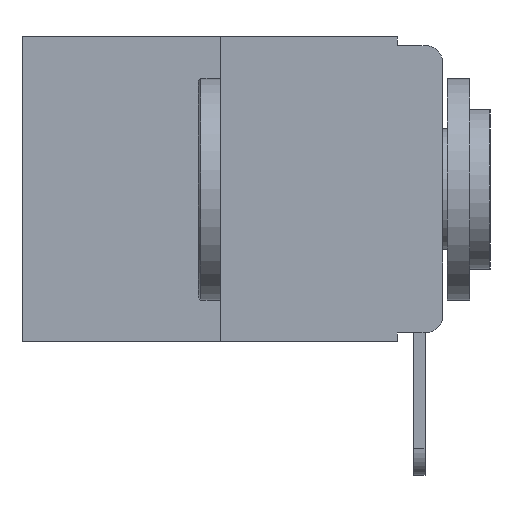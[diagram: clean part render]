
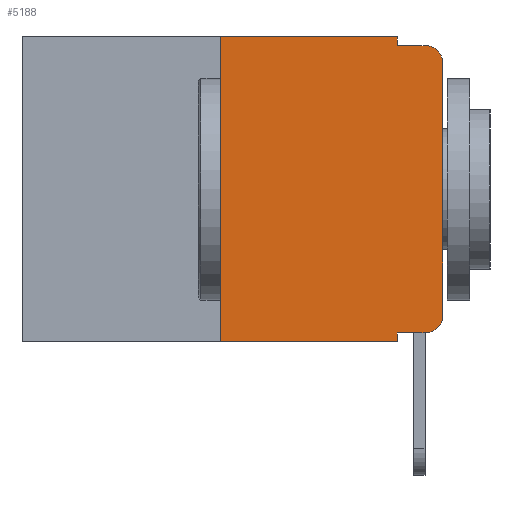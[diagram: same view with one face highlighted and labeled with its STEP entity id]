
A CAD part, left-side view. The second image highlights one B-rep face of the part: STEP entity #5188.
In plain terms, the highlighted planar face has unit normal (-1, 0, 0).
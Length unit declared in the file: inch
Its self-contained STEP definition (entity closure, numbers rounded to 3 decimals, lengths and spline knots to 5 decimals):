
#161 = ORIENTED_EDGE ( 'NONE', *, *, #17154, .T. ) ;
#173 = ORIENTED_EDGE ( 'NONE', *, *, #4821, .T. ) ;
#313 = DIRECTION ( 'NONE',  ( 0., 0., -1. ) ) ;
#349 = CARTESIAN_POINT ( 'NONE',  ( 0., 0.051, -0.343 ) ) ;
#486 = CARTESIAN_POINT ( 'NONE',  ( 0., 0.02, -0.01 ) ) ;
#583 = VECTOR ( 'NONE', #7805, 39.37008 ) ;
#1150 = ORIENTED_EDGE ( 'NONE', *, *, #4353, .F. ) ;
#1375 = CARTESIAN_POINT ( 'NONE',  ( 0., 0.02, -0.03 ) ) ;
#1557 = CARTESIAN_POINT ( 'NONE',  ( 0., 0., -0.313 ) ) ;
#2229 = CARTESIAN_POINT ( 'NONE',  ( 0., 0., 0. ) ) ;
#2324 = VERTEX_POINT ( 'NONE', #6563 ) ;
#2375 = CARTESIAN_POINT ( 'NONE',  ( 0., 0.473, -0.343 ) ) ;
#2437 = CARTESIAN_POINT ( 'NONE',  ( 0., 0.02, -0.333 ) ) ;
#2798 = ORIENTED_EDGE ( 'NONE', *, *, #17335, .T. ) ;
#2860 = PLANE ( 'NONE',  #12674 ) ;
#2863 = LINE ( 'NONE', #10259, #14258 ) ;
#2988 = ORIENTED_EDGE ( 'NONE', *, *, #12930, .T. ) ;
#3462 = DIRECTION ( 'NONE',  ( 0., -1., 0. ) ) ;
#3961 = VERTEX_POINT ( 'NONE', #7849 ) ;
#4121 = EDGE_CURVE ( 'NONE', #17209, #17401, #12028, .T. ) ;
#4143 = VECTOR ( 'NONE', #10056, 39.37008 ) ;
#4353 = EDGE_CURVE ( 'NONE', #2324, #9739, #11388, .T. ) ;
#4698 = VECTOR ( 'NONE', #7822, 39.37008 ) ;
#4821 = EDGE_CURVE ( 'NONE', #17401, #7610, #11574, .T. ) ;
#5105 = DIRECTION ( 'NONE',  ( 0., -1., 0. ) ) ;
#5109 = ORIENTED_EDGE ( 'NONE', *, *, #11330, .F. ) ;
#5188 = ADVANCED_FACE ( 'NONE', ( #11133 ), #2860, .F. ) ;
#5298 = EDGE_CURVE ( 'NONE', #9739, #8309, #14917, .T. ) ;
#5314 = DIRECTION ( 'NONE',  ( -1., 0., 0. ) ) ;
#5518 = VERTEX_POINT ( 'NONE', #8218 ) ;
#5855 = AXIS2_PLACEMENT_3D ( 'NONE', #8024, #13446, #9250 ) ;
#5874 = EDGE_CURVE ( 'NONE', #3961, #2324, #2863, .T. ) ;
#5970 = ORIENTED_EDGE ( 'NONE', *, *, #4121, .T. ) ;
#6563 = CARTESIAN_POINT ( 'NONE',  ( 0., 0.25, 0. ) ) ;
#7096 = ORIENTED_EDGE ( 'NONE', *, *, #5874, .F. ) ;
#7230 = CIRCLE ( 'NONE', #14387, 0.02 ) ;
#7289 = CARTESIAN_POINT ( 'NONE',  ( 0., 0.051, 0. ) ) ;
#7610 = VERTEX_POINT ( 'NONE', #8194 ) ;
#7805 = DIRECTION ( 'NONE',  ( 0., 0., 1. ) ) ;
#7822 = DIRECTION ( 'NONE',  ( 0., -1., 0. ) ) ;
#7849 = CARTESIAN_POINT ( 'NONE',  ( 0., 0.25, -0.343 ) ) ;
#7949 = ORIENTED_EDGE ( 'NONE', *, *, #11587, .F. ) ;
#8024 = CARTESIAN_POINT ( 'NONE',  ( 0., 0.02, -0.313 ) ) ;
#8194 = CARTESIAN_POINT ( 'NONE',  ( 0., 0., -0.03 ) ) ;
#8218 = CARTESIAN_POINT ( 'NONE',  ( 0., 0.051, -0.333 ) ) ;
#8309 = VERTEX_POINT ( 'NONE', #9450 ) ;
#8310 = LINE ( 'NONE', #2375, #4698 ) ;
#8541 = CARTESIAN_POINT ( 'NONE',  ( 0., 0.473, 0. ) ) ;
#9250 = DIRECTION ( 'NONE',  ( 0., 0., -1. ) ) ;
#9450 = CARTESIAN_POINT ( 'NONE',  ( 0., 0.051, -0.01 ) ) ;
#9498 = DIRECTION ( 'NONE',  ( 0., 0., -1. ) ) ;
#9739 = VERTEX_POINT ( 'NONE', #12941 ) ;
#9848 = ORIENTED_EDGE ( 'NONE', *, *, #5298, .F. ) ;
#10056 = DIRECTION ( 'NONE',  ( 0., 0., -1. ) ) ;
#10259 = CARTESIAN_POINT ( 'NONE',  ( 0., 0.25, 0. ) ) ;
#10479 = CARTESIAN_POINT ( 'NONE',  ( 0., 0.051, -0.333 ) ) ;
#10658 = DIRECTION ( 'NONE',  ( 0., 0., -1. ) ) ;
#10996 = VECTOR ( 'NONE', #10658, 39.37008 ) ;
#11133 = FACE_OUTER_BOUND ( 'NONE', #14471, .T. ) ;
#11330 = EDGE_CURVE ( 'NONE', #8309, #15200, #15468, .T. ) ;
#11385 = LINE ( 'NONE', #10479, #16628 ) ;
#11388 = LINE ( 'NONE', #8541, #14539 ) ;
#11574 = LINE ( 'NONE', #2229, #583 ) ;
#11587 = EDGE_CURVE ( 'NONE', #5518, #12744, #13545, .T. ) ;
#12028 = CIRCLE ( 'NONE', #5855, 0.02 ) ;
#12539 = DIRECTION ( 'NONE',  ( 1., 0., 0. ) ) ;
#12621 = DIRECTION ( 'NONE',  ( 0., -1., 0. ) ) ;
#12674 = AXIS2_PLACEMENT_3D ( 'NONE', #17414, #12539, #313 ) ;
#12744 = VERTEX_POINT ( 'NONE', #349 ) ;
#12930 = EDGE_CURVE ( 'NONE', #5518, #17209, #11385, .T. ) ;
#12941 = CARTESIAN_POINT ( 'NONE',  ( 0., 0.051, 0. ) ) ;
#13446 = DIRECTION ( 'NONE',  ( -1., 0., 0. ) ) ;
#13545 = LINE ( 'NONE', #14722, #10996 ) ;
#14173 = VECTOR ( 'NONE', #3462, 39.37008 ) ;
#14258 = VECTOR ( 'NONE', #17082, 39.37008 ) ;
#14387 = AXIS2_PLACEMENT_3D ( 'NONE', #1375, #5314, #9498 ) ;
#14471 = EDGE_LOOP ( 'NONE', ( #173, #2798, #5109, #9848, #1150, #7096, #161, #7949, #2988, #5970 ) ) ;
#14539 = VECTOR ( 'NONE', #12621, 39.37008 ) ;
#14722 = CARTESIAN_POINT ( 'NONE',  ( 0., 0.051, 0. ) ) ;
#14917 = LINE ( 'NONE', #7289, #4143 ) ;
#15200 = VERTEX_POINT ( 'NONE', #486 ) ;
#15468 = LINE ( 'NONE', #15677, #14173 ) ;
#15677 = CARTESIAN_POINT ( 'NONE',  ( 0., 0.051, -0.01 ) ) ;
#16628 = VECTOR ( 'NONE', #5105, 39.37008 ) ;
#17082 = DIRECTION ( 'NONE',  ( 0., 0., 1. ) ) ;
#17154 = EDGE_CURVE ( 'NONE', #3961, #12744, #8310, .T. ) ;
#17209 = VERTEX_POINT ( 'NONE', #2437 ) ;
#17335 = EDGE_CURVE ( 'NONE', #7610, #15200, #7230, .T. ) ;
#17401 = VERTEX_POINT ( 'NONE', #1557 ) ;
#17414 = CARTESIAN_POINT ( 'NONE',  ( 0., 0.473, 0. ) ) ;
